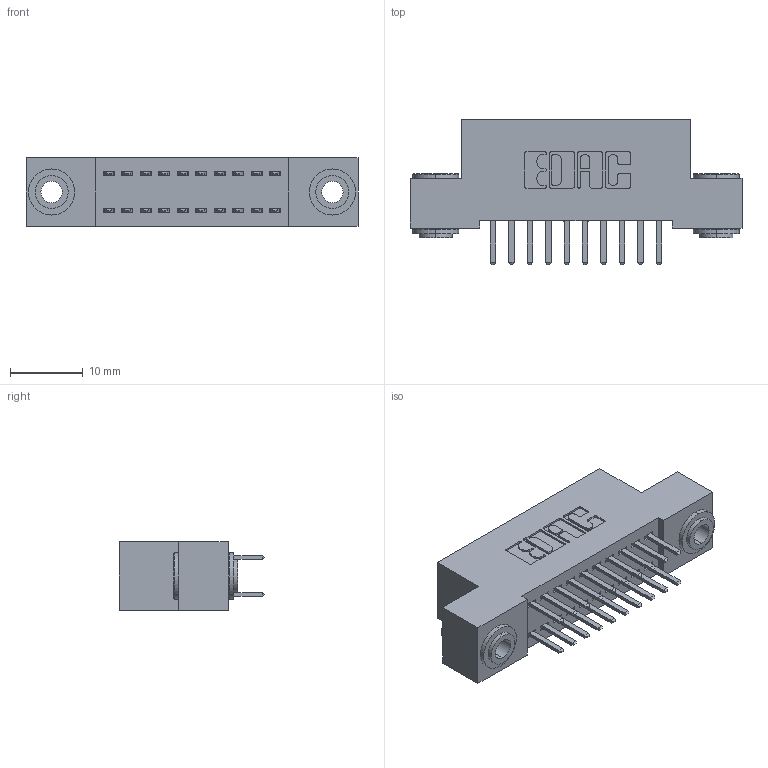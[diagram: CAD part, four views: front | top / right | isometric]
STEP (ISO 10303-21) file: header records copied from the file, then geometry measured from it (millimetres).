
FILE_DESCRIPTION (( 'STEP AP203' ), '1' );
FILE_NAME ('392-020-520-203.STEP', '2019-10-07T04:53:27', ( '' ), ( '' ), 'SwSTEP 2.0', 'SolidWorks 2016', '' );
FILE_SCHEMA (( 'CONFIG_CONTROL_DESIGN' ));
Length unit declared in the file: inch
Products named in the file (4): 345-292-001_345-293-120; 342-250-002_345-250-002-102; 392-020-520-203; 342 Part_.156 TH
Assembly tree (23 placements, depth 2):
  392-020-520-203
    342 Part_.156 TH
    345-292-001_345-293-120  x20
    342-250-002_345-250-002-102  x2
Bounding box: 45.72 x 20.02 x 9.4 mm (x, y, z)
Volume: 3970.5 mm3; surface area: 5867.8 mm2
Topology: 23 solids, 23 shells, 1268 faces, 3635 edges, 2366 vertices
Faces by surface type: plane 836, cylinder 424, cone 8
Entity records: 11204 total; most frequent: CARTESIAN_POINT 1881, ORIENTED_EDGE 1798, DIRECTION 1685, EDGE_CURVE 899, LINE 743, VECTOR 743, VERTEX_POINT 594, AXIS2_PLACEMENT_3D 471
